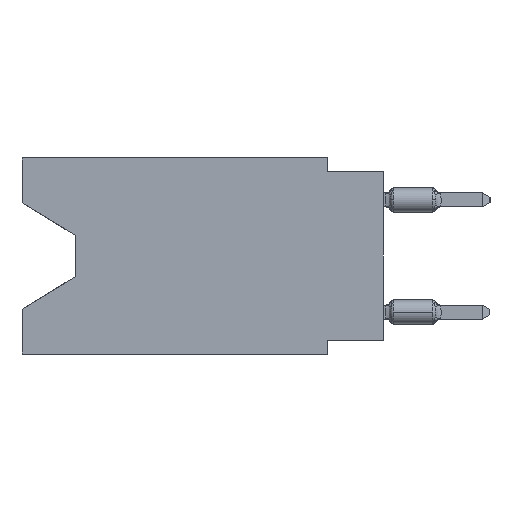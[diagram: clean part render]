
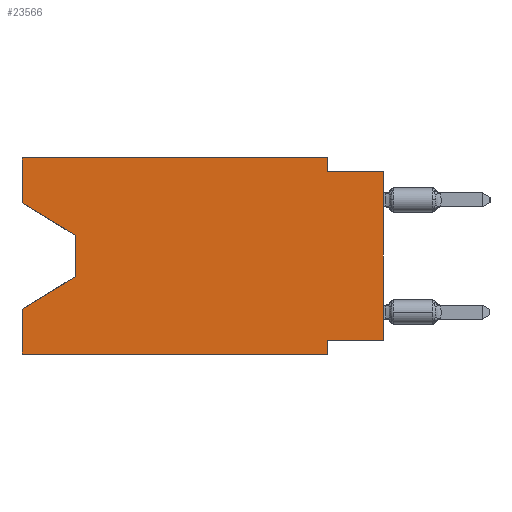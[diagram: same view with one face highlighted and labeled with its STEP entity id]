
A CAD part, left-side view. The second image highlights one B-rep face of the part: STEP entity #23566.
In plain terms, the highlighted planar face has unit normal (-1, 0, 0).
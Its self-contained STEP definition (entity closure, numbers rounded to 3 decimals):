
#281 = ORIENTED_EDGE ( 'NONE', *, *, #3344, .F. ) ;
#296 = VECTOR ( 'NONE', #17605, 1000. ) ;
#434 = DIRECTION ( 'NONE',  ( 0., -1., 0. ) ) ;
#554 = VERTEX_POINT ( 'NONE', #9696 ) ;
#643 = EDGE_CURVE ( 'NONE', #15391, #16338, #30974, .T. ) ;
#718 = VECTOR ( 'NONE', #25332, 1000. ) ;
#739 = DIRECTION ( 'NONE',  ( 0., -0.855, -0.519 ) ) ;
#1040 = VECTOR ( 'NONE', #739, 1000. ) ;
#1333 = DIRECTION ( 'NONE',  ( 0., 1., 0. ) ) ;
#1348 = VECTOR ( 'NONE', #29913, 1000. ) ;
#1872 = VERTEX_POINT ( 'NONE', #22578 ) ;
#2764 = VERTEX_POINT ( 'NONE', #31735 ) ;
#3344 = EDGE_CURVE ( 'NONE', #8009, #10538, #11704, .T. ) ;
#3368 = EDGE_CURVE ( 'NONE', #16338, #31856, #13059, .T. ) ;
#4931 = ORIENTED_EDGE ( 'NONE', *, *, #643, .T. ) ;
#5041 = DIRECTION ( 'NONE',  ( 1., 0., 0. ) ) ;
#5869 = CARTESIAN_POINT ( 'NONE',  ( 0., 16.383, -8.89 ) ) ;
#6693 = EDGE_CURVE ( 'NONE', #554, #15391, #22011, .T. ) ;
#6922 = CARTESIAN_POINT ( 'NONE',  ( 0., 0., -0.635 ) ) ;
#7245 = ORIENTED_EDGE ( 'NONE', *, *, #16980, .F. ) ;
#7444 = VECTOR ( 'NONE', #9519, 1000. ) ;
#7668 = CARTESIAN_POINT ( 'NONE',  ( 0., 2.54, -8.255 ) ) ;
#7732 = DIRECTION ( 'NONE',  ( 0., 0.855, -0.519 ) ) ;
#8009 = VERTEX_POINT ( 'NONE', #11584 ) ;
#8097 = CARTESIAN_POINT ( 'NONE',  ( 0., 2.54, -8.89 ) ) ;
#9419 = EDGE_CURVE ( 'NONE', #10538, #1872, #19998, .T. ) ;
#9519 = DIRECTION ( 'NONE',  ( 0., 0., -1. ) ) ;
#9633 = CARTESIAN_POINT ( 'NONE',  ( 0., 16.383, 0. ) ) ;
#9638 = DIRECTION ( 'NONE',  ( 0., 0., 1. ) ) ;
#9696 = CARTESIAN_POINT ( 'NONE',  ( 0., 16.383, -2.038 ) ) ;
#10538 = VERTEX_POINT ( 'NONE', #17613 ) ;
#10602 = ORIENTED_EDGE ( 'NONE', *, *, #20158, .T. ) ;
#10691 = ORIENTED_EDGE ( 'NONE', *, *, #3368, .T. ) ;
#11584 = CARTESIAN_POINT ( 'NONE',  ( 0., 16.383, 0. ) ) ;
#11704 = LINE ( 'NONE', #19435, #1348 ) ;
#11983 = ORIENTED_EDGE ( 'NONE', *, *, #9419, .F. ) ;
#12766 = PLANE ( 'NONE',  #24971 ) ;
#12839 = VECTOR ( 'NONE', #7732, 1000. ) ;
#12881 = CARTESIAN_POINT ( 'NONE',  ( 0., 16.383, 0. ) ) ;
#13059 = LINE ( 'NONE', #26266, #12839 ) ;
#14042 = VECTOR ( 'NONE', #19331, 1000. ) ;
#14445 = DIRECTION ( 'NONE',  ( 0., 0., 1. ) ) ;
#14648 = EDGE_CURVE ( 'NONE', #1872, #20689, #30497, .T. ) ;
#14685 = ORIENTED_EDGE ( 'NONE', *, *, #16776, .F. ) ;
#15260 = LINE ( 'NONE', #25725, #25084 ) ;
#15391 = VERTEX_POINT ( 'NONE', #32093 ) ;
#16338 = VERTEX_POINT ( 'NONE', #30455 ) ;
#16776 = EDGE_CURVE ( 'NONE', #26708, #31856, #27152, .T. ) ;
#16980 = EDGE_CURVE ( 'NONE', #2764, #18845, #27245, .T. ) ;
#17605 = DIRECTION ( 'NONE',  ( 0., 0., -1. ) ) ;
#17613 = CARTESIAN_POINT ( 'NONE',  ( 0., 2.54, 0. ) ) ;
#18572 = DIRECTION ( 'NONE',  ( 0., 0., -1. ) ) ;
#18623 = CARTESIAN_POINT ( 'NONE',  ( 0., 2.54, -8.89 ) ) ;
#18845 = VERTEX_POINT ( 'NONE', #7668 ) ;
#19182 = CARTESIAN_POINT ( 'NONE',  ( 0., 0., -8.255 ) ) ;
#19331 = DIRECTION ( 'NONE',  ( 0., 0., 1. ) ) ;
#19435 = CARTESIAN_POINT ( 'NONE',  ( 0., 16.383, 0. ) ) ;
#19998 = LINE ( 'NONE', #30651, #296 ) ;
#20158 = EDGE_CURVE ( 'NONE', #2764, #20689, #21739, .T. ) ;
#20689 = VERTEX_POINT ( 'NONE', #6922 ) ;
#21607 = EDGE_CURVE ( 'NONE', #26708, #27443, #15260, .T. ) ;
#21739 = LINE ( 'NONE', #27231, #14042 ) ;
#22011 = LINE ( 'NONE', #29570, #1040 ) ;
#22578 = CARTESIAN_POINT ( 'NONE',  ( 0., 2.54, -0.635 ) ) ;
#22839 = ORIENTED_EDGE ( 'NONE', *, *, #21607, .T. ) ;
#23025 = LINE ( 'NONE', #12881, #27668 ) ;
#23232 = CARTESIAN_POINT ( 'NONE',  ( 0., 16.383, 0. ) ) ;
#23407 = DIRECTION ( 'NONE',  ( 0., 0., -1. ) ) ;
#23566 = ADVANCED_FACE ( 'NONE', ( #31156 ), #12766, .F. ) ;
#24302 = VECTOR ( 'NONE', #18572, 1000. ) ;
#24829 = CARTESIAN_POINT ( 'NONE',  ( 0., 0., -0.635 ) ) ;
#24971 = AXIS2_PLACEMENT_3D ( 'NONE', #23232, #5041, #23407 ) ;
#25084 = VECTOR ( 'NONE', #434, 1000. ) ;
#25129 = VECTOR ( 'NONE', #1333, 1000. ) ;
#25332 = DIRECTION ( 'NONE',  ( 0., -1., 0. ) ) ;
#25725 = CARTESIAN_POINT ( 'NONE',  ( 0., 16.383, -8.89 ) ) ;
#26035 = EDGE_LOOP ( 'NONE', ( #27406, #4931, #10691, #14685, #22839, #28103, #7245, #10602, #32661, #11983, #281, #31753 ) ) ;
#26266 = CARTESIAN_POINT ( 'NONE',  ( 0., 13.97, -5.385 ) ) ;
#26708 = VERTEX_POINT ( 'NONE', #5869 ) ;
#27152 = LINE ( 'NONE', #9633, #27670 ) ;
#27231 = CARTESIAN_POINT ( 'NONE',  ( 0., 0., 0. ) ) ;
#27245 = LINE ( 'NONE', #19182, #25129 ) ;
#27406 = ORIENTED_EDGE ( 'NONE', *, *, #6693, .T. ) ;
#27443 = VERTEX_POINT ( 'NONE', #18623 ) ;
#27668 = VECTOR ( 'NONE', #9638, 1000. ) ;
#27670 = VECTOR ( 'NONE', #14445, 1000. ) ;
#28103 = ORIENTED_EDGE ( 'NONE', *, *, #31809, .F. ) ;
#28873 = LINE ( 'NONE', #8097, #24302 ) ;
#29570 = CARTESIAN_POINT ( 'NONE',  ( 0., 16.383, -2.038 ) ) ;
#29913 = DIRECTION ( 'NONE',  ( 0., -1., 0. ) ) ;
#30455 = CARTESIAN_POINT ( 'NONE',  ( 0., 13.97, -5.385 ) ) ;
#30497 = LINE ( 'NONE', #24829, #718 ) ;
#30651 = CARTESIAN_POINT ( 'NONE',  ( 0., 2.54, 0. ) ) ;
#30974 = LINE ( 'NONE', #33061, #7444 ) ;
#31156 = FACE_OUTER_BOUND ( 'NONE', #26035, .T. ) ;
#31735 = CARTESIAN_POINT ( 'NONE',  ( 0., 0., -8.255 ) ) ;
#31753 = ORIENTED_EDGE ( 'NONE', *, *, #33339, .F. ) ;
#31809 = EDGE_CURVE ( 'NONE', #18845, #27443, #28873, .T. ) ;
#31856 = VERTEX_POINT ( 'NONE', #32143 ) ;
#32093 = CARTESIAN_POINT ( 'NONE',  ( 0., 13.97, -3.505 ) ) ;
#32143 = CARTESIAN_POINT ( 'NONE',  ( 0., 16.383, -6.852 ) ) ;
#32661 = ORIENTED_EDGE ( 'NONE', *, *, #14648, .F. ) ;
#33061 = CARTESIAN_POINT ( 'NONE',  ( 0., 13.97, -3.505 ) ) ;
#33339 = EDGE_CURVE ( 'NONE', #554, #8009, #23025, .T. ) ;
